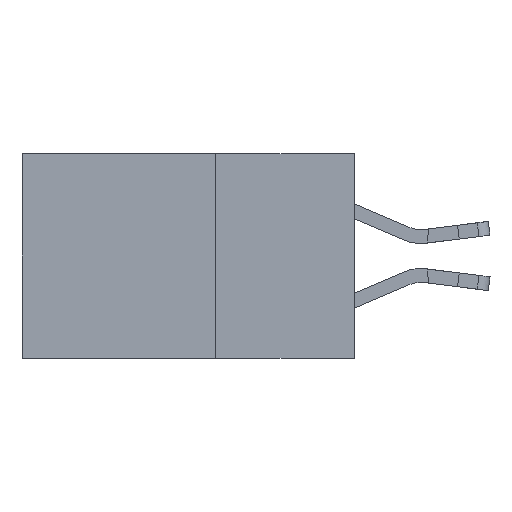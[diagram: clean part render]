
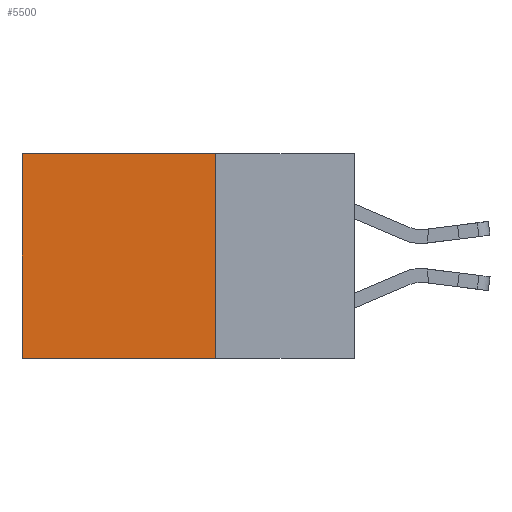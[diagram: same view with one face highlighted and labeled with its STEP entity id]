
A CAD part, left-side view. The second image highlights one B-rep face of the part: STEP entity #5500.
In plain terms, the highlighted planar face has unit normal (-1, 0, 0).
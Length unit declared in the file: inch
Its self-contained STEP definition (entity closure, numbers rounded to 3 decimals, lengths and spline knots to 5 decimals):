
#352 = CARTESIAN_POINT ( 'NONE',  ( 0.298, 0.25, 0. ) ) ;
#1368 = CARTESIAN_POINT ( 'NONE',  ( 0.298, 0.25, -0.37 ) ) ;
#1614 = VECTOR ( 'NONE', #8793, 39.37008 ) ;
#1947 = DIRECTION ( 'NONE',  ( 0., 0., -1. ) ) ;
#2117 = CARTESIAN_POINT ( 'NONE',  ( 0.298, 0.25, 0. ) ) ;
#2391 = ORIENTED_EDGE ( 'NONE', *, *, #3340, .F. ) ;
#2913 = ORIENTED_EDGE ( 'NONE', *, *, #12849, .T. ) ;
#3302 = EDGE_CURVE ( 'NONE', #8049, #17221, #10375, .T. ) ;
#3340 = EDGE_CURVE ( 'NONE', #8925, #8049, #5830, .T. ) ;
#4024 = VECTOR ( 'NONE', #17185, 39.37008 ) ;
#5500 = ADVANCED_FACE ( 'NONE', ( #15222 ), #11359, .F. ) ;
#5830 = LINE ( 'NONE', #2117, #1614 ) ;
#6445 = DIRECTION ( 'NONE',  ( 0., 1., 0. ) ) ;
#6514 = CARTESIAN_POINT ( 'NONE',  ( 0.298, 0.25, -0.37 ) ) ;
#7243 = CARTESIAN_POINT ( 'NONE',  ( 0.298, 0.6, -0.37 ) ) ;
#7779 = AXIS2_PLACEMENT_3D ( 'NONE', #352, #11515, #1947 ) ;
#8049 = VERTEX_POINT ( 'NONE', #1368 ) ;
#8793 = DIRECTION ( 'NONE',  ( 0., 0., -1. ) ) ;
#8925 = VERTEX_POINT ( 'NONE', #14280 ) ;
#9256 = LINE ( 'NONE', #20366, #4024 ) ;
#9365 = VECTOR ( 'NONE', #6445, 39.37008 ) ;
#9865 = CARTESIAN_POINT ( 'NONE',  ( 0.298, 0.25, 0. ) ) ;
#10365 = VECTOR ( 'NONE', #12963, 39.37008 ) ;
#10375 = LINE ( 'NONE', #6514, #9365 ) ;
#11359 = PLANE ( 'NONE',  #7779 ) ;
#11515 = DIRECTION ( 'NONE',  ( 1., 0., 0. ) ) ;
#12849 = EDGE_CURVE ( 'NONE', #19233, #17221, #9256, .T. ) ;
#12963 = DIRECTION ( 'NONE',  ( 0., 1., 0. ) ) ;
#13537 = ORIENTED_EDGE ( 'NONE', *, *, #3302, .F. ) ;
#14280 = CARTESIAN_POINT ( 'NONE',  ( 0.298, 0.25, 0. ) ) ;
#14641 = LINE ( 'NONE', #9865, #10365 ) ;
#15222 = FACE_OUTER_BOUND ( 'NONE', #18110, .T. ) ;
#17185 = DIRECTION ( 'NONE',  ( 0., 0., -1. ) ) ;
#17221 = VERTEX_POINT ( 'NONE', #7243 ) ;
#18110 = EDGE_LOOP ( 'NONE', ( #2913, #13537, #2391, #20536 ) ) ;
#18194 = CARTESIAN_POINT ( 'NONE',  ( 0.298, 0.6, 0. ) ) ;
#18916 = EDGE_CURVE ( 'NONE', #8925, #19233, #14641, .T. ) ;
#19233 = VERTEX_POINT ( 'NONE', #18194 ) ;
#20366 = CARTESIAN_POINT ( 'NONE',  ( 0.298, 0.6, 0. ) ) ;
#20536 = ORIENTED_EDGE ( 'NONE', *, *, #18916, .T. ) ;
